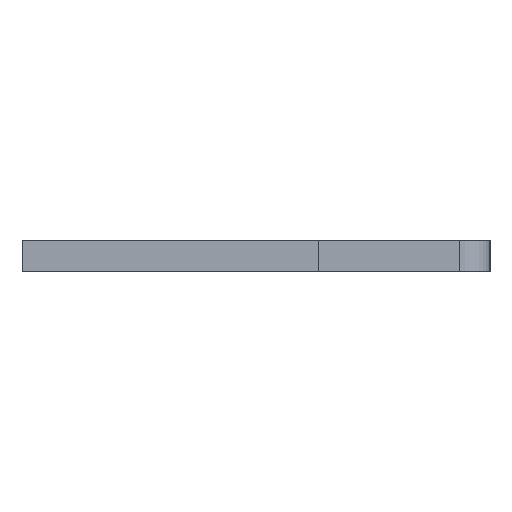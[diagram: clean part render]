
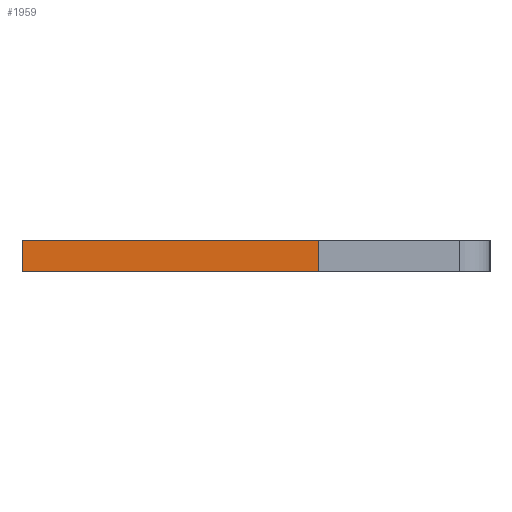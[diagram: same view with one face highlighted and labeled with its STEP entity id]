
A CAD part, left-side view. The second image highlights one B-rep face of the part: STEP entity #1959.
In plain terms, the highlighted face is planar.
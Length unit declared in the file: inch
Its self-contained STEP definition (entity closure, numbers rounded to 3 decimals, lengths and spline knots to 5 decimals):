
#4 = EDGE_CURVE ( 'NONE', #79, #1086, #2761, .T. ) ;
#49 = EDGE_CURVE ( 'NONE', #1330, #79, #1189, .T. ) ;
#79 = VERTEX_POINT ( 'NONE', #2090 ) ;
#141 = FACE_OUTER_BOUND ( 'NONE', #544, .T. ) ;
#159 = DIRECTION ( 'NONE',  ( 0., 1., 0. ) ) ;
#219 = CARTESIAN_POINT ( 'NONE',  ( -0.01, -0.04, -0.04 ) ) ;
#343 = PLANE ( 'NONE',  #1143 ) ;
#517 = CARTESIAN_POINT ( 'NONE',  ( -0.01, 0.15, -0.04 ) ) ;
#544 = EDGE_LOOP ( 'NONE', ( #1571, #1558, #585, #1987 ) ) ;
#572 = CARTESIAN_POINT ( 'NONE',  ( -0.01, 0.15, -0.04 ) ) ;
#585 = ORIENTED_EDGE ( 'NONE', *, *, #49, .F. ) ;
#731 = VECTOR ( 'NONE', #2897, 39.37008 ) ;
#871 = LINE ( 'NONE', #572, #731 ) ;
#1086 = VERTEX_POINT ( 'NONE', #517 ) ;
#1114 = VECTOR ( 'NONE', #159, 39.37008 ) ;
#1143 = AXIS2_PLACEMENT_3D ( 'NONE', #2474, #2248, #1748 ) ;
#1189 = LINE ( 'NONE', #1342, #1114 ) ;
#1330 = VERTEX_POINT ( 'NONE', #2188 ) ;
#1342 = CARTESIAN_POINT ( 'NONE',  ( 0.01, 0.15, -0.04 ) ) ;
#1528 = VECTOR ( 'NONE', #1841, 39.37008 ) ;
#1558 = ORIENTED_EDGE ( 'NONE', *, *, #4, .F. ) ;
#1571 = ORIENTED_EDGE ( 'NONE', *, *, #1845, .T. ) ;
#1616 = VECTOR ( 'NONE', #2793, 39.37008 ) ;
#1748 = DIRECTION ( 'NONE',  ( 1., 0., 0. ) ) ;
#1841 = DIRECTION ( 'NONE',  ( -1., 0., 0. ) ) ;
#1845 = EDGE_CURVE ( 'NONE', #2732, #1086, #871, .T. ) ;
#1959 = ADVANCED_FACE ( 'NONE', ( #141 ), #343, .F. ) ;
#1987 = ORIENTED_EDGE ( 'NONE', *, *, #2589, .T. ) ;
#2090 = CARTESIAN_POINT ( 'NONE',  ( 0.01, 0.15, -0.04 ) ) ;
#2188 = CARTESIAN_POINT ( 'NONE',  ( 0.01, -0.04, -0.04 ) ) ;
#2248 = DIRECTION ( 'NONE',  ( 0., 0., 1. ) ) ;
#2308 = CARTESIAN_POINT ( 'NONE',  ( 0.01, -0.04, -0.04 ) ) ;
#2474 = CARTESIAN_POINT ( 'NONE',  ( 0.01, 0.15, -0.04 ) ) ;
#2521 = CARTESIAN_POINT ( 'NONE',  ( 0.01, 0.15, -0.04 ) ) ;
#2536 = LINE ( 'NONE', #2308, #1616 ) ;
#2589 = EDGE_CURVE ( 'NONE', #1330, #2732, #2536, .T. ) ;
#2732 = VERTEX_POINT ( 'NONE', #219 ) ;
#2761 = LINE ( 'NONE', #2521, #1528 ) ;
#2793 = DIRECTION ( 'NONE',  ( -1., 0., 0. ) ) ;
#2897 = DIRECTION ( 'NONE',  ( 0., 1., 0. ) ) ;
